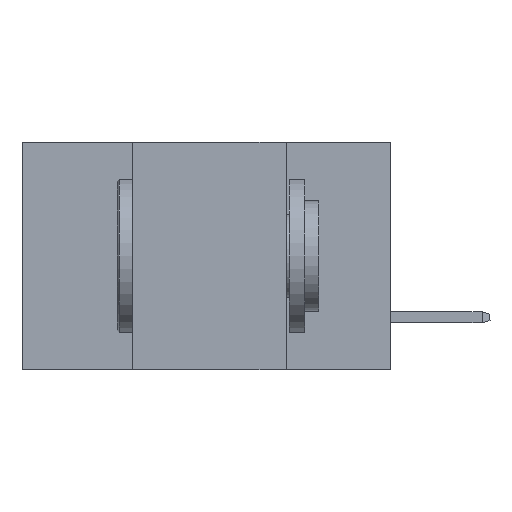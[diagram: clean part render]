
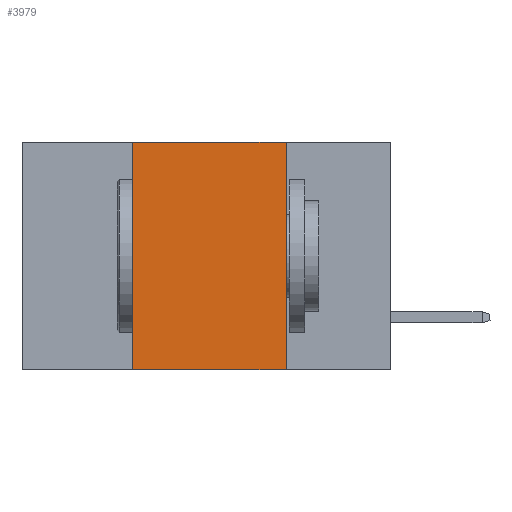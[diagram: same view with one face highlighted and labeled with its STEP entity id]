
A CAD part, left-side view. The second image highlights one B-rep face of the part: STEP entity #3979.
In plain terms, the highlighted planar face has unit normal (-1, 0, 0).
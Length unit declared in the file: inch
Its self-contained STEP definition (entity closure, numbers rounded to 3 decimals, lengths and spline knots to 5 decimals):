
#274 = EDGE_CURVE ( 'NONE', #6490, #10485, #12135, .T. ) ;
#1064 = DIRECTION ( 'NONE',  ( 1., 0., 0. ) ) ;
#1998 = ORIENTED_EDGE ( 'NONE', *, *, #4215, .F. ) ;
#2687 = ORIENTED_EDGE ( 'NONE', *, *, #6015, .T. ) ;
#2773 = ORIENTED_EDGE ( 'NONE', *, *, #6500, .F. ) ;
#3034 = VERTEX_POINT ( 'NONE', #13383 ) ;
#3935 = ORIENTED_EDGE ( 'NONE', *, *, #274, .F. ) ;
#3979 = ADVANCED_FACE ( 'NONE', ( #11545 ), #7229, .F. ) ;
#4215 = EDGE_CURVE ( 'NONE', #10485, #3034, #12110, .T. ) ;
#4305 = DIRECTION ( 'NONE',  ( 0., 0., -1. ) ) ;
#4734 = CARTESIAN_POINT ( 'NONE',  ( 0., 0.6, 0. ) ) ;
#4803 = DIRECTION ( 'NONE',  ( 0., 0., -1. ) ) ;
#4874 = VECTOR ( 'NONE', #7355, 39.37008 ) ;
#5209 = LINE ( 'NONE', #10433, #8836 ) ;
#6015 = EDGE_CURVE ( 'NONE', #6490, #8720, #6720, .T. ) ;
#6490 = VERTEX_POINT ( 'NONE', #15294 ) ;
#6500 = EDGE_CURVE ( 'NONE', #3034, #8720, #5209, .T. ) ;
#6586 = CARTESIAN_POINT ( 'NONE',  ( 0., 0.17, -0.37 ) ) ;
#6720 = LINE ( 'NONE', #14164, #9782 ) ;
#6929 = DIRECTION ( 'NONE',  ( 0., -1., 0. ) ) ;
#7229 = PLANE ( 'NONE',  #13159 ) ;
#7355 = DIRECTION ( 'NONE',  ( 0., -1., 0. ) ) ;
#8720 = VERTEX_POINT ( 'NONE', #6586 ) ;
#8836 = VECTOR ( 'NONE', #4305, 39.37008 ) ;
#8984 = DIRECTION ( 'NONE',  ( 0., 0., 1. ) ) ;
#9779 = CARTESIAN_POINT ( 'NONE',  ( 0., 0.42, 0. ) ) ;
#9782 = VECTOR ( 'NONE', #6929, 39.37008 ) ;
#10433 = CARTESIAN_POINT ( 'NONE',  ( 0., 0.17, 0. ) ) ;
#10485 = VERTEX_POINT ( 'NONE', #11518 ) ;
#11518 = CARTESIAN_POINT ( 'NONE',  ( 0., 0.42, 0. ) ) ;
#11545 = FACE_OUTER_BOUND ( 'NONE', #13060, .T. ) ;
#11952 = VECTOR ( 'NONE', #8984, 39.37008 ) ;
#12087 = CARTESIAN_POINT ( 'NONE',  ( 0., 0.6, 0. ) ) ;
#12110 = LINE ( 'NONE', #4734, #4874 ) ;
#12135 = LINE ( 'NONE', #9779, #11952 ) ;
#13060 = EDGE_LOOP ( 'NONE', ( #2773, #1998, #3935, #2687 ) ) ;
#13159 = AXIS2_PLACEMENT_3D ( 'NONE', #12087, #1064, #4803 ) ;
#13383 = CARTESIAN_POINT ( 'NONE',  ( 0., 0.17, 0. ) ) ;
#14164 = CARTESIAN_POINT ( 'NONE',  ( 0., 0.6, -0.37 ) ) ;
#15294 = CARTESIAN_POINT ( 'NONE',  ( 0., 0.42, -0.37 ) ) ;
